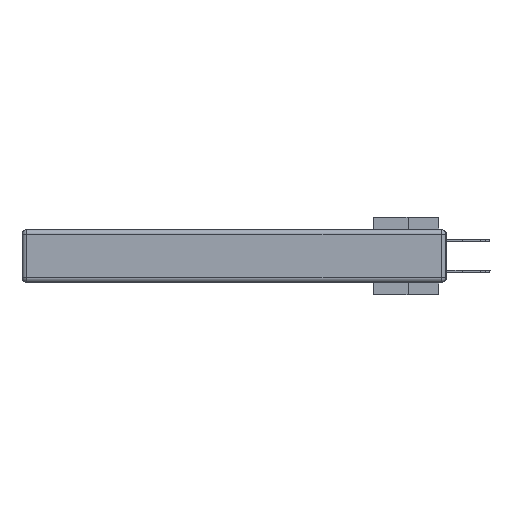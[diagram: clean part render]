
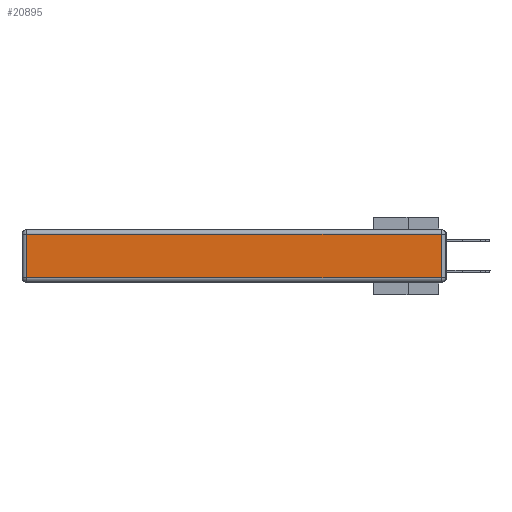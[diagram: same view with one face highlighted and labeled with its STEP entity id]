
A CAD part, left-side view. The second image highlights one B-rep face of the part: STEP entity #20895.
In plain terms, the highlighted planar face has unit normal (-1, 0, 0).
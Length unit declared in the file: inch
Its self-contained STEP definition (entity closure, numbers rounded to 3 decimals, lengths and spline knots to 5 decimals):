
#776 = LINE ( 'NONE', #30550, #20360 ) ;
#1342 = CARTESIAN_POINT ( 'NONE',  ( 0., 2.72, -0.313 ) ) ;
#3466 = EDGE_CURVE ( 'NONE', #33099, #20650, #17810, .T. ) ;
#4436 = EDGE_LOOP ( 'NONE', ( #28438, #25409, #8138, #16581 ) ) ;
#4572 = DIRECTION ( 'NONE',  ( 0., 0., -1. ) ) ;
#5694 = DIRECTION ( 'NONE',  ( 0., -1., 0. ) ) ;
#5866 = EDGE_CURVE ( 'NONE', #20650, #21999, #19648, .T. ) ;
#7867 = AXIS2_PLACEMENT_3D ( 'NONE', #22668, #15071, #15181 ) ;
#8138 = ORIENTED_EDGE ( 'NONE', *, *, #14359, .T. ) ;
#8625 = VERTEX_POINT ( 'NONE', #23725 ) ;
#10167 = EDGE_CURVE ( 'NONE', #21999, #8625, #776, .T. ) ;
#11142 = CARTESIAN_POINT ( 'NONE',  ( 0., 2.75, -0.03 ) ) ;
#11383 = VECTOR ( 'NONE', #13715, 39.37008 ) ;
#12487 = PLANE ( 'NONE',  #7867 ) ;
#13715 = DIRECTION ( 'NONE',  ( 0., 1., 0. ) ) ;
#14359 = EDGE_CURVE ( 'NONE', #8625, #33099, #22211, .T. ) ;
#14598 = CARTESIAN_POINT ( 'NONE',  ( 0., 2.72, -0.343 ) ) ;
#15071 = DIRECTION ( 'NONE',  ( -1., 0., 0. ) ) ;
#15181 = DIRECTION ( 'NONE',  ( 0., 0., 1. ) ) ;
#15435 = CARTESIAN_POINT ( 'NONE',  ( 0., 2.72, -0.03 ) ) ;
#15832 = CARTESIAN_POINT ( 'NONE',  ( 0., 0., -0.313 ) ) ;
#16581 = ORIENTED_EDGE ( 'NONE', *, *, #3466, .T. ) ;
#17007 = VECTOR ( 'NONE', #4572, 39.37008 ) ;
#17810 = LINE ( 'NONE', #14598, #17007 ) ;
#19648 = LINE ( 'NONE', #15832, #23669 ) ;
#20360 = VECTOR ( 'NONE', #33059, 39.37008 ) ;
#20650 = VERTEX_POINT ( 'NONE', #1342 ) ;
#20895 = ADVANCED_FACE ( 'NONE', ( #22383 ), #12487, .T. ) ;
#21999 = VERTEX_POINT ( 'NONE', #31001 ) ;
#22211 = LINE ( 'NONE', #11142, #11383 ) ;
#22383 = FACE_OUTER_BOUND ( 'NONE', #4436, .T. ) ;
#22668 = CARTESIAN_POINT ( 'NONE',  ( 0., 0., -0.343 ) ) ;
#23669 = VECTOR ( 'NONE', #5694, 39.37008 ) ;
#23725 = CARTESIAN_POINT ( 'NONE',  ( 0., 0.03, -0.03 ) ) ;
#25409 = ORIENTED_EDGE ( 'NONE', *, *, #10167, .T. ) ;
#28438 = ORIENTED_EDGE ( 'NONE', *, *, #5866, .T. ) ;
#30550 = CARTESIAN_POINT ( 'NONE',  ( 0., 0.03, -0.343 ) ) ;
#31001 = CARTESIAN_POINT ( 'NONE',  ( 0., 0.03, -0.313 ) ) ;
#33059 = DIRECTION ( 'NONE',  ( 0., 0., 1. ) ) ;
#33099 = VERTEX_POINT ( 'NONE', #15435 ) ;
